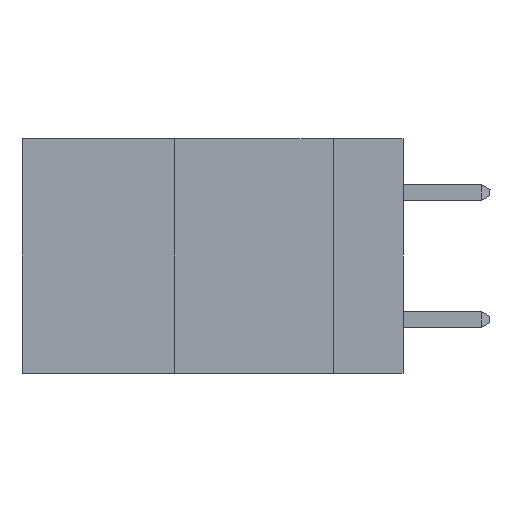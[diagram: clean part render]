
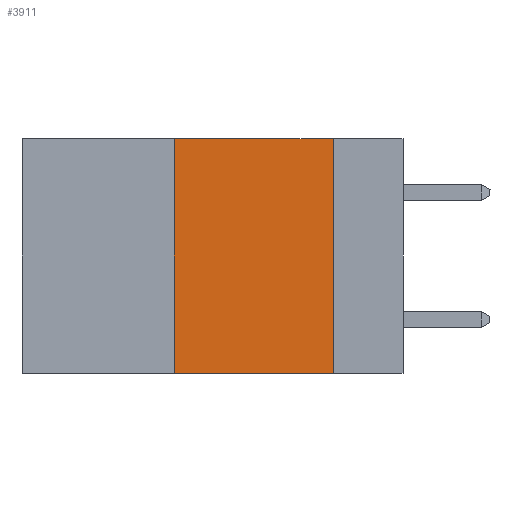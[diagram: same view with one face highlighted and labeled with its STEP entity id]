
A CAD part, left-side view. The second image highlights one B-rep face of the part: STEP entity #3911.
In plain terms, the highlighted planar face has unit normal (-1, 0, 0).
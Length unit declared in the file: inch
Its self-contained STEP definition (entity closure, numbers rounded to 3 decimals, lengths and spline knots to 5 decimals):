
#119 = PLANE ( 'NONE',  #12568 ) ;
#408 = CARTESIAN_POINT ( 'NONE',  ( 0., 0.6, 0. ) ) ;
#895 = LINE ( 'NONE', #7486, #3617 ) ;
#1226 = CARTESIAN_POINT ( 'NONE',  ( 0., 0.36, 0. ) ) ;
#1881 = EDGE_CURVE ( 'NONE', #6111, #5931, #7956, .T. ) ;
#1997 = CARTESIAN_POINT ( 'NONE',  ( 0., 0.11, 0. ) ) ;
#2466 = ORIENTED_EDGE ( 'NONE', *, *, #8955, .T. ) ;
#2966 = ORIENTED_EDGE ( 'NONE', *, *, #8658, .F. ) ;
#2979 = ORIENTED_EDGE ( 'NONE', *, *, #1881, .F. ) ;
#3617 = VECTOR ( 'NONE', #8445, 39.37008 ) ;
#3755 = ORIENTED_EDGE ( 'NONE', *, *, #7681, .F. ) ;
#3911 = ADVANCED_FACE ( 'NONE', ( #7999 ), #119, .F. ) ;
#4912 = LINE ( 'NONE', #7555, #9778 ) ;
#5357 = DIRECTION ( 'NONE',  ( 0., -1., 0. ) ) ;
#5931 = VERTEX_POINT ( 'NONE', #1997 ) ;
#5971 = DIRECTION ( 'NONE',  ( 0., -1., 0. ) ) ;
#6111 = VERTEX_POINT ( 'NONE', #1226 ) ;
#7486 = CARTESIAN_POINT ( 'NONE',  ( 0., 0.11, 0. ) ) ;
#7555 = CARTESIAN_POINT ( 'NONE',  ( 0., 0.36, 0. ) ) ;
#7628 = DIRECTION ( 'NONE',  ( 0., 0., -1. ) ) ;
#7681 = EDGE_CURVE ( 'NONE', #5931, #8137, #895, .T. ) ;
#7914 = CARTESIAN_POINT ( 'NONE',  ( 0., 0.6, -0.37 ) ) ;
#7930 = CARTESIAN_POINT ( 'NONE',  ( 0., 0.11, -0.37 ) ) ;
#7956 = LINE ( 'NONE', #10572, #12244 ) ;
#7999 = FACE_OUTER_BOUND ( 'NONE', #12430, .T. ) ;
#8137 = VERTEX_POINT ( 'NONE', #7930 ) ;
#8445 = DIRECTION ( 'NONE',  ( 0., 0., -1. ) ) ;
#8513 = DIRECTION ( 'NONE',  ( 0., 0., 1. ) ) ;
#8533 = DIRECTION ( 'NONE',  ( 1., 0., 0. ) ) ;
#8658 = EDGE_CURVE ( 'NONE', #9853, #6111, #4912, .T. ) ;
#8955 = EDGE_CURVE ( 'NONE', #9853, #8137, #9917, .T. ) ;
#9778 = VECTOR ( 'NONE', #8513, 39.37008 ) ;
#9853 = VERTEX_POINT ( 'NONE', #11498 ) ;
#9917 = LINE ( 'NONE', #7914, #12001 ) ;
#10572 = CARTESIAN_POINT ( 'NONE',  ( 0., 0.6, 0. ) ) ;
#11498 = CARTESIAN_POINT ( 'NONE',  ( 0., 0.36, -0.37 ) ) ;
#12001 = VECTOR ( 'NONE', #5971, 39.37008 ) ;
#12244 = VECTOR ( 'NONE', #5357, 39.37008 ) ;
#12430 = EDGE_LOOP ( 'NONE', ( #3755, #2979, #2966, #2466 ) ) ;
#12568 = AXIS2_PLACEMENT_3D ( 'NONE', #408, #8533, #7628 ) ;
